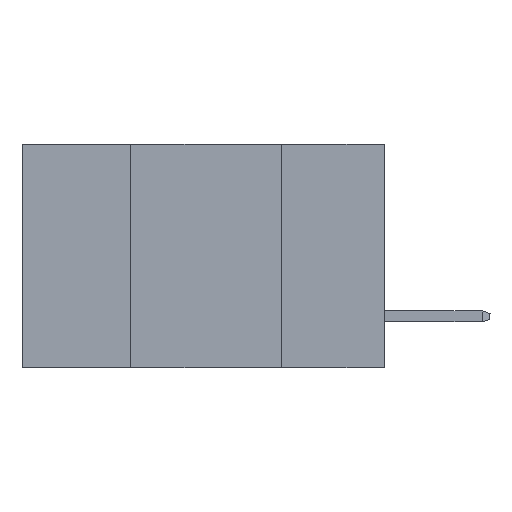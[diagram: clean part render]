
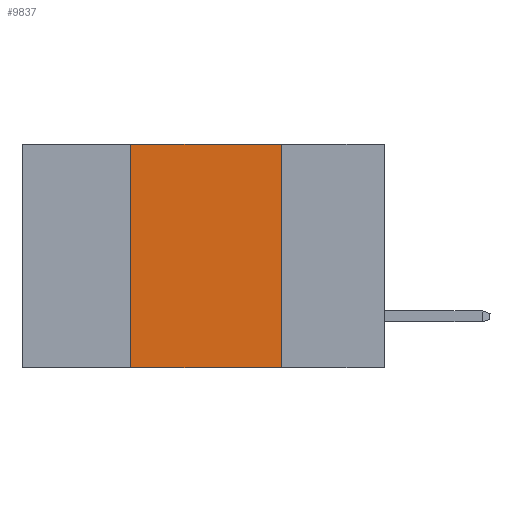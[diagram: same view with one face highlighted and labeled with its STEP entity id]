
A CAD part, left-side view. The second image highlights one B-rep face of the part: STEP entity #9837.
In plain terms, the highlighted planar face has unit normal (-1, 0, 0).
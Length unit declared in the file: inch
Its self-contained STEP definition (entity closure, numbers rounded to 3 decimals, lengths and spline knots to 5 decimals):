
#39 = CARTESIAN_POINT ( 'NONE',  ( 0., 0.6, 0. ) ) ;
#246 = CARTESIAN_POINT ( 'NONE',  ( 0., 0.6, -0.37 ) ) ;
#256 = VECTOR ( 'NONE', #750, 39.37008 ) ;
#261 = LINE ( 'NONE', #3309, #10313 ) ;
#614 = ORIENTED_EDGE ( 'NONE', *, *, #7426, .T. ) ;
#615 = VERTEX_POINT ( 'NONE', #2548 ) ;
#750 = DIRECTION ( 'NONE',  ( 0., 0., 1. ) ) ;
#1359 = EDGE_CURVE ( 'NONE', #615, #9450, #7005, .T. ) ;
#1632 = CARTESIAN_POINT ( 'NONE',  ( 0., 0.6, 0. ) ) ;
#1838 = EDGE_CURVE ( 'NONE', #9450, #5370, #261, .T. ) ;
#2059 = DIRECTION ( 'NONE',  ( 0., -1., 0. ) ) ;
#2548 = CARTESIAN_POINT ( 'NONE',  ( 0., 0.42, 0. ) ) ;
#2662 = VERTEX_POINT ( 'NONE', #11251 ) ;
#3234 = DIRECTION ( 'NONE',  ( 0., 0., -1. ) ) ;
#3247 = AXIS2_PLACEMENT_3D ( 'NONE', #1632, #8814, #5390 ) ;
#3309 = CARTESIAN_POINT ( 'NONE',  ( 0., 0.17, -0.37 ) ) ;
#3950 = CARTESIAN_POINT ( 'NONE',  ( 0., 0.17, 0. ) ) ;
#4241 = LINE ( 'NONE', #246, #8820 ) ;
#4303 = FACE_OUTER_BOUND ( 'NONE', #11628, .T. ) ;
#4683 = PLANE ( 'NONE',  #3247 ) ;
#4820 = CARTESIAN_POINT ( 'NONE',  ( 0., 0.42, -0.37 ) ) ;
#5263 = DIRECTION ( 'NONE',  ( 0., -1., 0. ) ) ;
#5370 = VERTEX_POINT ( 'NONE', #7739 ) ;
#5390 = DIRECTION ( 'NONE',  ( 0., 0., -1. ) ) ;
#6161 = ORIENTED_EDGE ( 'NONE', *, *, #1359, .F. ) ;
#6722 = LINE ( 'NONE', #4820, #256 ) ;
#7005 = LINE ( 'NONE', #39, #8937 ) ;
#7426 = EDGE_CURVE ( 'NONE', #2662, #5370, #4241, .T. ) ;
#7739 = CARTESIAN_POINT ( 'NONE',  ( 0., 0.17, -0.37 ) ) ;
#8333 = ORIENTED_EDGE ( 'NONE', *, *, #1838, .F. ) ;
#8814 = DIRECTION ( 'NONE',  ( 1., 0., 0. ) ) ;
#8820 = VECTOR ( 'NONE', #5263, 39.37008 ) ;
#8937 = VECTOR ( 'NONE', #2059, 39.37008 ) ;
#9450 = VERTEX_POINT ( 'NONE', #3950 ) ;
#9837 = ADVANCED_FACE ( 'NONE', ( #4303 ), #4683, .F. ) ;
#10313 = VECTOR ( 'NONE', #3234, 39.37008 ) ;
#11251 = CARTESIAN_POINT ( 'NONE',  ( 0., 0.42, -0.37 ) ) ;
#11390 = ORIENTED_EDGE ( 'NONE', *, *, #11752, .F. ) ;
#11628 = EDGE_LOOP ( 'NONE', ( #8333, #6161, #11390, #614 ) ) ;
#11752 = EDGE_CURVE ( 'NONE', #2662, #615, #6722, .T. ) ;
